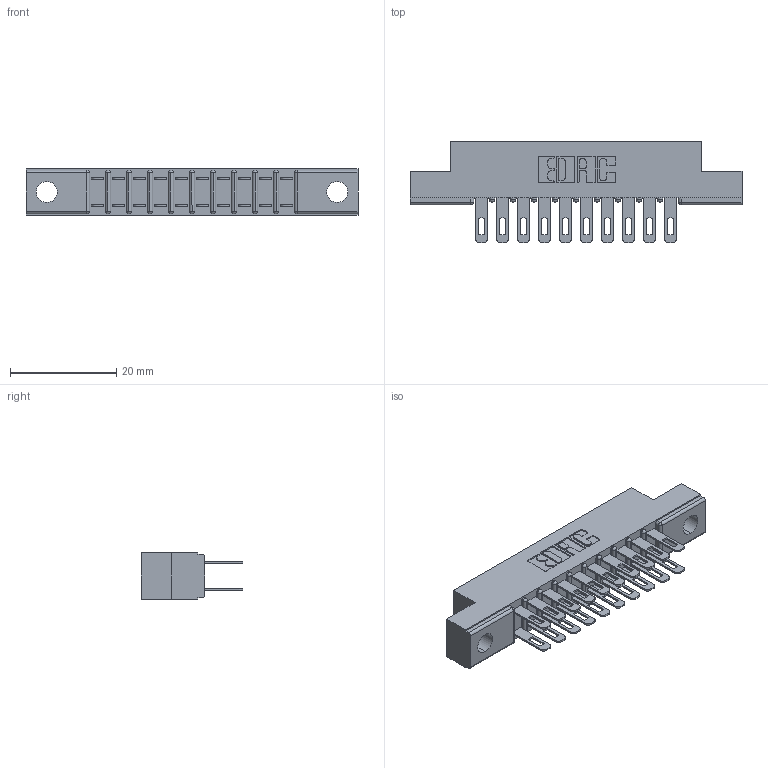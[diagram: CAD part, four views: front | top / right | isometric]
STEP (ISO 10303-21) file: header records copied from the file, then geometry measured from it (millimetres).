
FILE_DESCRIPTION (( 'STEP AP203' ), '1' );
FILE_NAME ('357-020-500-204.STEP', '2019-09-17T20:17:18', ( '' ), ( '' ), 'SwSTEP 2.0', 'SolidWorks 2016', '' );
FILE_SCHEMA (( 'CONFIG_CONTROL_DESIGN' ));
Length unit declared in the file: inch
Products named in the file (3): 307 Part_.156 Dia Mounting Holes; 307-290-001_500; 357-020-500-204
Assembly tree (21 placements, depth 2):
  357-020-500-204
    307 Part_.156 Dia Mounting Holes
    307-290-001_500  x20
Bounding box: 62.64 x 19.18 x 8.71 mm (x, y, z)
Volume: 4049.8 mm3; surface area: 6733.5 mm2
Topology: 21 solids, 21 shells, 1063 faces, 2959 edges, 1914 vertices
Faces by surface type: plane 684, cylinder 357, sphere 22
Entity records: 13230 total; most frequent: CARTESIAN_POINT 2176, ORIENTED_EDGE 2150, DIRECTION 2139, EDGE_CURVE 1075, LINE 817, VECTOR 817, VERTEX_POINT 698, AXIS2_PLACEMENT_3D 661
